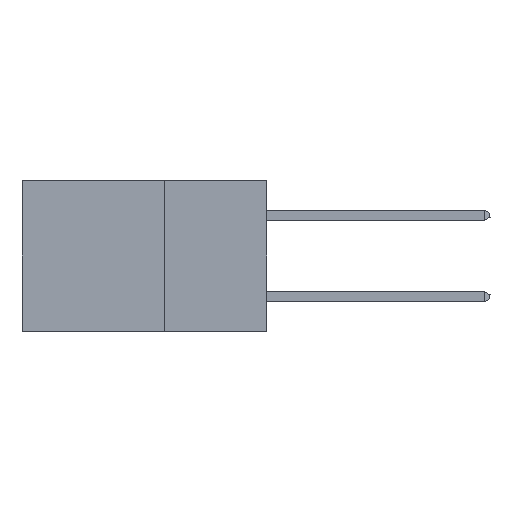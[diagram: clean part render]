
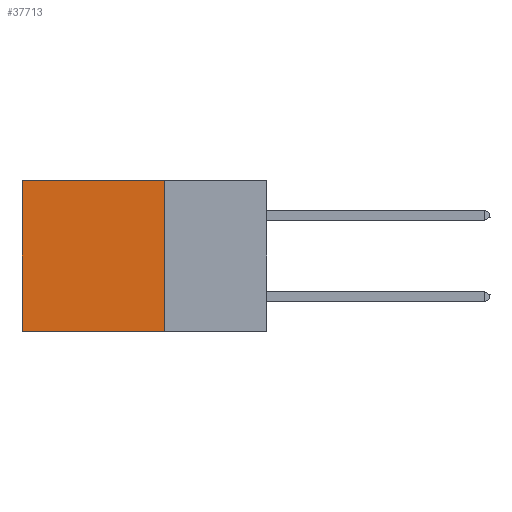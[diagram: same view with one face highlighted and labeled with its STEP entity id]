
A CAD part, left-side view. The second image highlights one B-rep face of the part: STEP entity #37713.
In plain terms, the highlighted planar face has unit normal (-1, 0, 0).
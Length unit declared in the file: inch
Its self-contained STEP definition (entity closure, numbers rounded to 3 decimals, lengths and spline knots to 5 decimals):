
#1085 = EDGE_LOOP ( 'NONE', ( #5745, #30076, #39790, #38595 ) ) ;
#1795 = LINE ( 'NONE', #44433, #33019 ) ;
#2445 = VERTEX_POINT ( 'NONE', #25478 ) ;
#2568 = DIRECTION ( 'NONE',  ( 0., 0., -1. ) ) ;
#4440 = EDGE_CURVE ( 'NONE', #6704, #44166, #1795, .T. ) ;
#5443 = AXIS2_PLACEMENT_3D ( 'NONE', #13003, #41698, #2568 ) ;
#5745 = ORIENTED_EDGE ( 'NONE', *, *, #15993, .T. ) ;
#5970 = DIRECTION ( 'NONE',  ( 0., 0., -1. ) ) ;
#6453 = VECTOR ( 'NONE', #24780, 39.37008 ) ;
#6704 = VERTEX_POINT ( 'NONE', #21346 ) ;
#7760 = CARTESIAN_POINT ( 'NONE',  ( 0.2875, 0.6, -0.37 ) ) ;
#10851 = CARTESIAN_POINT ( 'NONE',  ( 0.2875, 0.25, -0.37 ) ) ;
#13003 = CARTESIAN_POINT ( 'NONE',  ( 0.2875, 0.25, 0. ) ) ;
#15993 = EDGE_CURVE ( 'NONE', #2445, #17209, #36459, .T. ) ;
#17209 = VERTEX_POINT ( 'NONE', #7760 ) ;
#17388 = LINE ( 'NONE', #24336, #6453 ) ;
#18862 = DIRECTION ( 'NONE',  ( 0., 0., -1. ) ) ;
#21346 = CARTESIAN_POINT ( 'NONE',  ( 0.2875, 0.25, 0. ) ) ;
#21440 = EDGE_CURVE ( 'NONE', #44166, #17209, #27749, .T. ) ;
#24336 = CARTESIAN_POINT ( 'NONE',  ( 0.2875, 0.25, 0. ) ) ;
#24780 = DIRECTION ( 'NONE',  ( 0., 1., 0. ) ) ;
#25478 = CARTESIAN_POINT ( 'NONE',  ( 0.2875, 0.6, 0. ) ) ;
#26582 = VECTOR ( 'NONE', #28199, 39.37008 ) ;
#27559 = PLANE ( 'NONE',  #5443 ) ;
#27749 = LINE ( 'NONE', #10851, #26582 ) ;
#27829 = VECTOR ( 'NONE', #18862, 39.37008 ) ;
#28199 = DIRECTION ( 'NONE',  ( 0., 1., 0. ) ) ;
#30076 = ORIENTED_EDGE ( 'NONE', *, *, #21440, .F. ) ;
#30212 = EDGE_CURVE ( 'NONE', #6704, #2445, #17388, .T. ) ;
#32749 = CARTESIAN_POINT ( 'NONE',  ( 0.2875, 0.6, 0. ) ) ;
#33019 = VECTOR ( 'NONE', #5970, 39.37008 ) ;
#34290 = FACE_OUTER_BOUND ( 'NONE', #1085, .T. ) ;
#36459 = LINE ( 'NONE', #32749, #27829 ) ;
#37713 = ADVANCED_FACE ( 'NONE', ( #34290 ), #27559, .F. ) ;
#38595 = ORIENTED_EDGE ( 'NONE', *, *, #30212, .T. ) ;
#39790 = ORIENTED_EDGE ( 'NONE', *, *, #4440, .F. ) ;
#41698 = DIRECTION ( 'NONE',  ( 1., 0., 0. ) ) ;
#43351 = CARTESIAN_POINT ( 'NONE',  ( 0.2875, 0.25, -0.37 ) ) ;
#44166 = VERTEX_POINT ( 'NONE', #43351 ) ;
#44433 = CARTESIAN_POINT ( 'NONE',  ( 0.2875, 0.25, 0. ) ) ;
